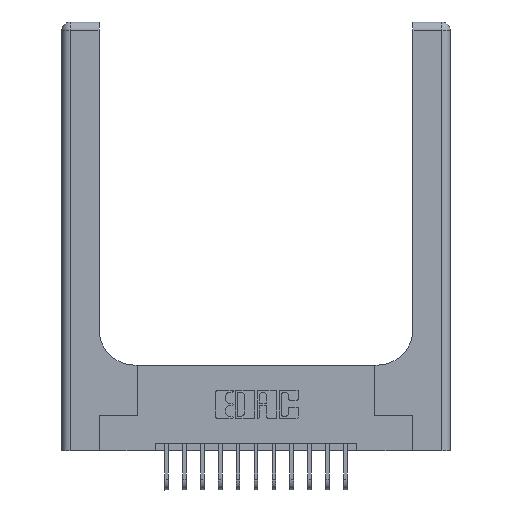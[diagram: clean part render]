
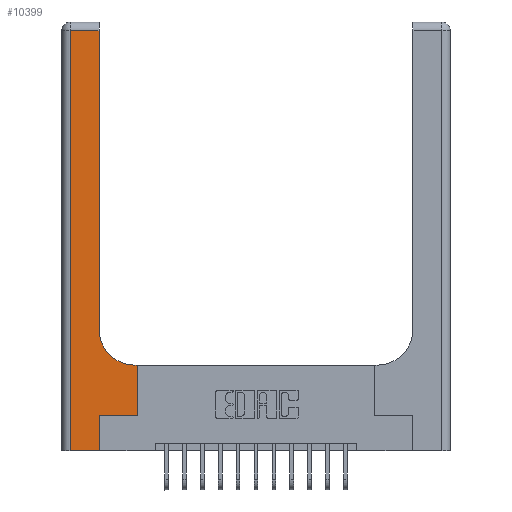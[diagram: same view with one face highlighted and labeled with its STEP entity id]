
A CAD part, top view. The second image highlights one B-rep face of the part: STEP entity #10399.
In plain terms, the highlighted planar face has unit normal (0, 0, 1).
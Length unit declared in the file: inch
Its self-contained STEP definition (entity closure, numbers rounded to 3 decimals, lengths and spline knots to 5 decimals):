
#8 = LINE ( 'NONE', #8770, #8635 ) ;
#179 = CARTESIAN_POINT ( 'NONE',  ( 0.06, 0., 0.37 ) ) ;
#424 = CARTESIAN_POINT ( 'NONE',  ( 0.26, 0.85, 0.37 ) ) ;
#811 = CARTESIAN_POINT ( 'NONE',  ( 0.51, 0.85, 0.37 ) ) ;
#823 = VERTEX_POINT ( 'NONE', #10099 ) ;
#1487 = LINE ( 'NONE', #5341, #2989 ) ;
#1552 = LINE ( 'NONE', #11842, #14037 ) ;
#2378 = DIRECTION ( 'NONE',  ( -1., 0., 0. ) ) ;
#2401 = DIRECTION ( 'NONE',  ( 0., 0., -1. ) ) ;
#2656 = VERTEX_POINT ( 'NONE', #7292 ) ;
#2701 = CIRCLE ( 'NONE', #4605, 0.25 ) ;
#2989 = VECTOR ( 'NONE', #5438, 39.37008 ) ;
#3356 = CARTESIAN_POINT ( 'NONE',  ( 0.06, 3., 0.37 ) ) ;
#3394 = EDGE_CURVE ( 'NONE', #11952, #13073, #8, .T. ) ;
#3522 = VECTOR ( 'NONE', #9771, 39.37008 ) ;
#4043 = CARTESIAN_POINT ( 'NONE',  ( 0., 2.94, 0.37 ) ) ;
#4051 = EDGE_CURVE ( 'NONE', #13844, #11571, #14916, .T. ) ;
#4250 = ORIENTED_EDGE ( 'NONE', *, *, #9855, .T. ) ;
#4304 = VERTEX_POINT ( 'NONE', #15323 ) ;
#4605 = AXIS2_PLACEMENT_3D ( 'NONE', #811, #2401, #4934 ) ;
#4709 = LINE ( 'NONE', #9844, #7026 ) ;
#4925 = EDGE_LOOP ( 'NONE', ( #16050, #12027, #5216, #14763, #7482, #7248, #10812, #16265, #4250 ) ) ;
#4934 = DIRECTION ( 'NONE',  ( 1., 0., 0. ) ) ;
#5216 = ORIENTED_EDGE ( 'NONE', *, *, #4051, .T. ) ;
#5228 = CARTESIAN_POINT ( 'NONE',  ( 0.06, 2.94, 0.37 ) ) ;
#5341 = CARTESIAN_POINT ( 'NONE',  ( 0.265, 0.25, 0.37 ) ) ;
#5438 = DIRECTION ( 'NONE',  ( 1., 0., 0. ) ) ;
#5975 = LINE ( 'NONE', #9689, #13186 ) ;
#6090 = EDGE_CURVE ( 'NONE', #15206, #2656, #8903, .T. ) ;
#6819 = DIRECTION ( 'NONE',  ( -1., 0., 0. ) ) ;
#7026 = VECTOR ( 'NONE', #12496, 39.37008 ) ;
#7248 = ORIENTED_EDGE ( 'NONE', *, *, #16689, .T. ) ;
#7292 = CARTESIAN_POINT ( 'NONE',  ( 0.26, 2.94, 0.37 ) ) ;
#7482 = ORIENTED_EDGE ( 'NONE', *, *, #8993, .T. ) ;
#7745 = LINE ( 'NONE', #4043, #9711 ) ;
#8014 = PLANE ( 'NONE',  #14869 ) ;
#8635 = VECTOR ( 'NONE', #2378, 39.37008 ) ;
#8770 = CARTESIAN_POINT ( 'NONE',  ( 0.26, 0.6, 0.37 ) ) ;
#8903 = LINE ( 'NONE', #10102, #9949 ) ;
#8993 = EDGE_CURVE ( 'NONE', #10603, #823, #5975, .T. ) ;
#9557 = CARTESIAN_POINT ( 'NONE',  ( 0.51, 0.6, 0.37 ) ) ;
#9689 = CARTESIAN_POINT ( 'NONE',  ( 0.265, 0., 0.37 ) ) ;
#9702 = CARTESIAN_POINT ( 'NONE',  ( 0.265, 0., 0.37 ) ) ;
#9706 = CARTESIAN_POINT ( 'NONE',  ( 0.528, 0.6, 0.37 ) ) ;
#9711 = VECTOR ( 'NONE', #6819, 39.37008 ) ;
#9771 = DIRECTION ( 'NONE',  ( 0., -1., 0. ) ) ;
#9844 = CARTESIAN_POINT ( 'NONE',  ( 0.528, 0.25, 0.37 ) ) ;
#9855 = EDGE_CURVE ( 'NONE', #13073, #15206, #2701, .T. ) ;
#9949 = VECTOR ( 'NONE', #16523, 39.37008 ) ;
#10099 = CARTESIAN_POINT ( 'NONE',  ( 0.265, 0.25, 0.37 ) ) ;
#10102 = CARTESIAN_POINT ( 'NONE',  ( 0.26, 3., 0.37 ) ) ;
#10399 = ADVANCED_FACE ( 'NONE', ( #15975 ), #8014, .F. ) ;
#10603 = VERTEX_POINT ( 'NONE', #9702 ) ;
#10742 = CARTESIAN_POINT ( 'NONE',  ( 0., 3., 0.37 ) ) ;
#10812 = ORIENTED_EDGE ( 'NONE', *, *, #15588, .T. ) ;
#10980 = DIRECTION ( 'NONE',  ( 0., 1., 0. ) ) ;
#11571 = VERTEX_POINT ( 'NONE', #179 ) ;
#11842 = CARTESIAN_POINT ( 'NONE',  ( 0., 0., 0.37 ) ) ;
#11952 = VERTEX_POINT ( 'NONE', #9706 ) ;
#12027 = ORIENTED_EDGE ( 'NONE', *, *, #15246, .T. ) ;
#12496 = DIRECTION ( 'NONE',  ( 0., 1., 0. ) ) ;
#13073 = VERTEX_POINT ( 'NONE', #9557 ) ;
#13186 = VECTOR ( 'NONE', #10980, 39.37008 ) ;
#13297 = DIRECTION ( 'NONE',  ( 0., 0., -1. ) ) ;
#13844 = VERTEX_POINT ( 'NONE', #5228 ) ;
#14037 = VECTOR ( 'NONE', #14626, 39.37008 ) ;
#14626 = DIRECTION ( 'NONE',  ( 1., 0., 0. ) ) ;
#14739 = EDGE_CURVE ( 'NONE', #11571, #10603, #1552, .T. ) ;
#14763 = ORIENTED_EDGE ( 'NONE', *, *, #14739, .T. ) ;
#14869 = AXIS2_PLACEMENT_3D ( 'NONE', #10742, #13297, #15803 ) ;
#14916 = LINE ( 'NONE', #3356, #3522 ) ;
#15206 = VERTEX_POINT ( 'NONE', #424 ) ;
#15246 = EDGE_CURVE ( 'NONE', #2656, #13844, #7745, .T. ) ;
#15323 = CARTESIAN_POINT ( 'NONE',  ( 0.528, 0.25, 0.37 ) ) ;
#15588 = EDGE_CURVE ( 'NONE', #4304, #11952, #4709, .T. ) ;
#15803 = DIRECTION ( 'NONE',  ( -1., 0., 0. ) ) ;
#15975 = FACE_OUTER_BOUND ( 'NONE', #4925, .T. ) ;
#16050 = ORIENTED_EDGE ( 'NONE', *, *, #6090, .T. ) ;
#16265 = ORIENTED_EDGE ( 'NONE', *, *, #3394, .T. ) ;
#16523 = DIRECTION ( 'NONE',  ( 0., 1., 0. ) ) ;
#16689 = EDGE_CURVE ( 'NONE', #823, #4304, #1487, .T. ) ;
